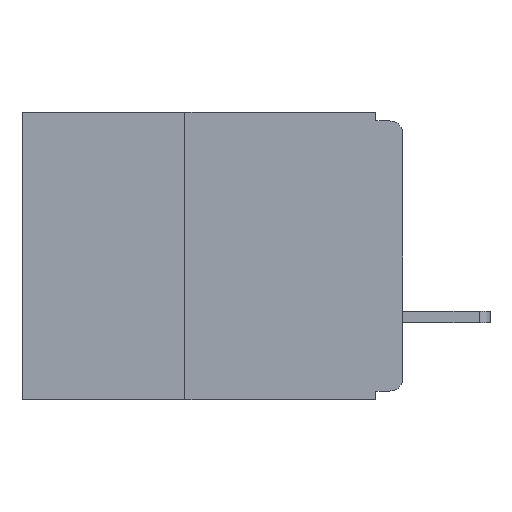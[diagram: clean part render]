
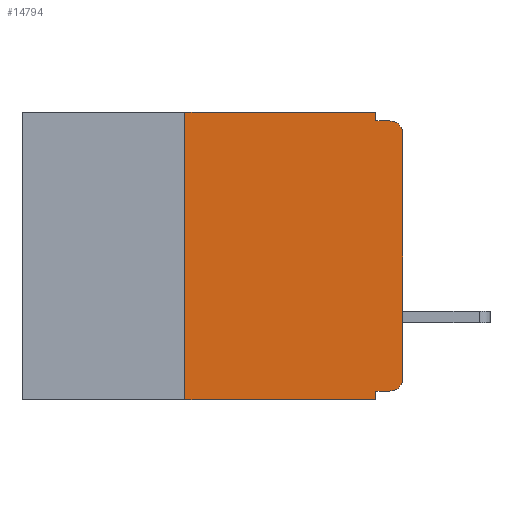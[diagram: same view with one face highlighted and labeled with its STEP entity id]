
A CAD part, left-side view. The second image highlights one B-rep face of the part: STEP entity #14794.
In plain terms, the highlighted planar face has unit normal (-1, 0, 0).
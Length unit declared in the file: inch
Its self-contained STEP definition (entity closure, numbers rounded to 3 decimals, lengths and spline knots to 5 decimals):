
#27 = CARTESIAN_POINT ( 'NONE',  ( 0., 0.015, -0.025 ) ) ;
#228 = CARTESIAN_POINT ( 'NONE',  ( 0., 0.031, -0.01 ) ) ;
#360 = DIRECTION ( 'NONE',  ( 0., 1., 0. ) ) ;
#453 = VERTEX_POINT ( 'NONE', #13101 ) ;
#534 = DIRECTION ( 'NONE',  ( 0., 0., -1. ) ) ;
#558 = ORIENTED_EDGE ( 'NONE', *, *, #16494, .F. ) ;
#812 = AXIS2_PLACEMENT_3D ( 'NONE', #17601, #11987, #534 ) ;
#1047 = CARTESIAN_POINT ( 'NONE',  ( 0., 0.031, 0. ) ) ;
#1176 = FACE_OUTER_BOUND ( 'NONE', #14192, .T. ) ;
#1273 = LINE ( 'NONE', #9878, #14703 ) ;
#1367 = CARTESIAN_POINT ( 'NONE',  ( 0., 0.015, -0.305 ) ) ;
#1764 = LINE ( 'NONE', #7067, #21351 ) ;
#1784 = ORIENTED_EDGE ( 'NONE', *, *, #13176, .T. ) ;
#1823 = EDGE_CURVE ( 'NONE', #15928, #16834, #15234, .T. ) ;
#1936 = DIRECTION ( 'NONE',  ( 0., 0., -1. ) ) ;
#3324 = DIRECTION ( 'NONE',  ( 0., 0., -1. ) ) ;
#3728 = EDGE_CURVE ( 'NONE', #16834, #7061, #1764, .T. ) ;
#4291 = DIRECTION ( 'NONE',  ( 0., -1., 0. ) ) ;
#4338 = LINE ( 'NONE', #4878, #9385 ) ;
#4878 = CARTESIAN_POINT ( 'NONE',  ( 0., 0.031, -0.33 ) ) ;
#5849 = LINE ( 'NONE', #16493, #15343 ) ;
#6194 = VERTEX_POINT ( 'NONE', #7119 ) ;
#6820 = ORIENTED_EDGE ( 'NONE', *, *, #11032, .F. ) ;
#7061 = VERTEX_POINT ( 'NONE', #9977 ) ;
#7067 = CARTESIAN_POINT ( 'NONE',  ( 0., 0., -0.01 ) ) ;
#7119 = CARTESIAN_POINT ( 'NONE',  ( 0., 0., -0.025 ) ) ;
#7645 = EDGE_CURVE ( 'NONE', #453, #6194, #23679, .T. ) ;
#8464 = AXIS2_PLACEMENT_3D ( 'NONE', #1367, #14717, #3324 ) ;
#8524 = ORIENTED_EDGE ( 'NONE', *, *, #1823, .F. ) ;
#9046 = ORIENTED_EDGE ( 'NONE', *, *, #3728, .F. ) ;
#9068 = ORIENTED_EDGE ( 'NONE', *, *, #16139, .T. ) ;
#9189 = VERTEX_POINT ( 'NONE', #18830 ) ;
#9385 = VECTOR ( 'NONE', #18143, 39.37008 ) ;
#9546 = ORIENTED_EDGE ( 'NONE', *, *, #7645, .T. ) ;
#9878 = CARTESIAN_POINT ( 'NONE',  ( 0., 0., -0.32 ) ) ;
#9977 = CARTESIAN_POINT ( 'NONE',  ( 0., 0.015, -0.01 ) ) ;
#10003 = ORIENTED_EDGE ( 'NONE', *, *, #20937, .T. ) ;
#10025 = EDGE_CURVE ( 'NONE', #9189, #18140, #4338, .T. ) ;
#10056 = PLANE ( 'NONE',  #812 ) ;
#10062 = VERTEX_POINT ( 'NONE', #16289 ) ;
#10843 = CARTESIAN_POINT ( 'NONE',  ( 0., 0.015, -0.32 ) ) ;
#11032 = EDGE_CURVE ( 'NONE', #23305, #9189, #1273, .T. ) ;
#11220 = VECTOR ( 'NONE', #16389, 39.37008 ) ;
#11987 = DIRECTION ( 'NONE',  ( 1., 0., 0. ) ) ;
#12233 = LINE ( 'NONE', #15660, #18452 ) ;
#13101 = CARTESIAN_POINT ( 'NONE',  ( 0., 0., -0.305 ) ) ;
#13176 = EDGE_CURVE ( 'NONE', #23305, #453, #18532, .T. ) ;
#13355 = DIRECTION ( 'NONE',  ( -1., 0., 0. ) ) ;
#13621 = DIRECTION ( 'NONE',  ( 0., 0., 1. ) ) ;
#13702 = VECTOR ( 'NONE', #13621, 39.37008 ) ;
#14192 = EDGE_LOOP ( 'NONE', ( #9546, #9068, #9046, #8524, #18566, #558, #10003, #19446, #6820, #1784 ) ) ;
#14532 = CARTESIAN_POINT ( 'NONE',  ( 0., 0.031, 0. ) ) ;
#14703 = VECTOR ( 'NONE', #360, 39.37008 ) ;
#14717 = DIRECTION ( 'NONE',  ( -1., 0., 0. ) ) ;
#14794 = ADVANCED_FACE ( 'NONE', ( #1176 ), #10056, .F. ) ;
#15234 = LINE ( 'NONE', #1047, #19674 ) ;
#15343 = VECTOR ( 'NONE', #18427, 39.37008 ) ;
#15428 = CARTESIAN_POINT ( 'NONE',  ( 0., 0., 0. ) ) ;
#15523 = AXIS2_PLACEMENT_3D ( 'NONE', #27, #13355, #1936 ) ;
#15660 = CARTESIAN_POINT ( 'NONE',  ( 0., 0.437, 0. ) ) ;
#15928 = VERTEX_POINT ( 'NONE', #14532 ) ;
#16139 = EDGE_CURVE ( 'NONE', #6194, #7061, #24498, .T. ) ;
#16289 = CARTESIAN_POINT ( 'NONE',  ( 0., 0.25, -0.33 ) ) ;
#16389 = DIRECTION ( 'NONE',  ( 0., 0., 1. ) ) ;
#16493 = CARTESIAN_POINT ( 'NONE',  ( 0., 0.437, -0.33 ) ) ;
#16494 = EDGE_CURVE ( 'NONE', #10062, #20219, #21258, .T. ) ;
#16834 = VERTEX_POINT ( 'NONE', #228 ) ;
#17601 = CARTESIAN_POINT ( 'NONE',  ( 0., 0.437, 0. ) ) ;
#18140 = VERTEX_POINT ( 'NONE', #23083 ) ;
#18143 = DIRECTION ( 'NONE',  ( 0., 0., -1. ) ) ;
#18427 = DIRECTION ( 'NONE',  ( 0., -1., 0. ) ) ;
#18440 = CARTESIAN_POINT ( 'NONE',  ( 0., 0.25, 0. ) ) ;
#18452 = VECTOR ( 'NONE', #4291, 39.37008 ) ;
#18532 = CIRCLE ( 'NONE', #8464, 0.015 ) ;
#18566 = ORIENTED_EDGE ( 'NONE', *, *, #18761, .F. ) ;
#18761 = EDGE_CURVE ( 'NONE', #20219, #15928, #12233, .T. ) ;
#18830 = CARTESIAN_POINT ( 'NONE',  ( 0., 0.031, -0.32 ) ) ;
#19446 = ORIENTED_EDGE ( 'NONE', *, *, #10025, .F. ) ;
#19674 = VECTOR ( 'NONE', #24501, 39.37008 ) ;
#20202 = CARTESIAN_POINT ( 'NONE',  ( 0., 0.25, -0.33 ) ) ;
#20219 = VERTEX_POINT ( 'NONE', #18440 ) ;
#20937 = EDGE_CURVE ( 'NONE', #10062, #18140, #5849, .T. ) ;
#21258 = LINE ( 'NONE', #20202, #11220 ) ;
#21351 = VECTOR ( 'NONE', #22255, 39.37008 ) ;
#22255 = DIRECTION ( 'NONE',  ( 0., -1., 0. ) ) ;
#23083 = CARTESIAN_POINT ( 'NONE',  ( 0., 0.031, -0.33 ) ) ;
#23305 = VERTEX_POINT ( 'NONE', #10843 ) ;
#23679 = LINE ( 'NONE', #15428, #13702 ) ;
#24498 = CIRCLE ( 'NONE', #15523, 0.015 ) ;
#24501 = DIRECTION ( 'NONE',  ( 0., 0., -1. ) ) ;
